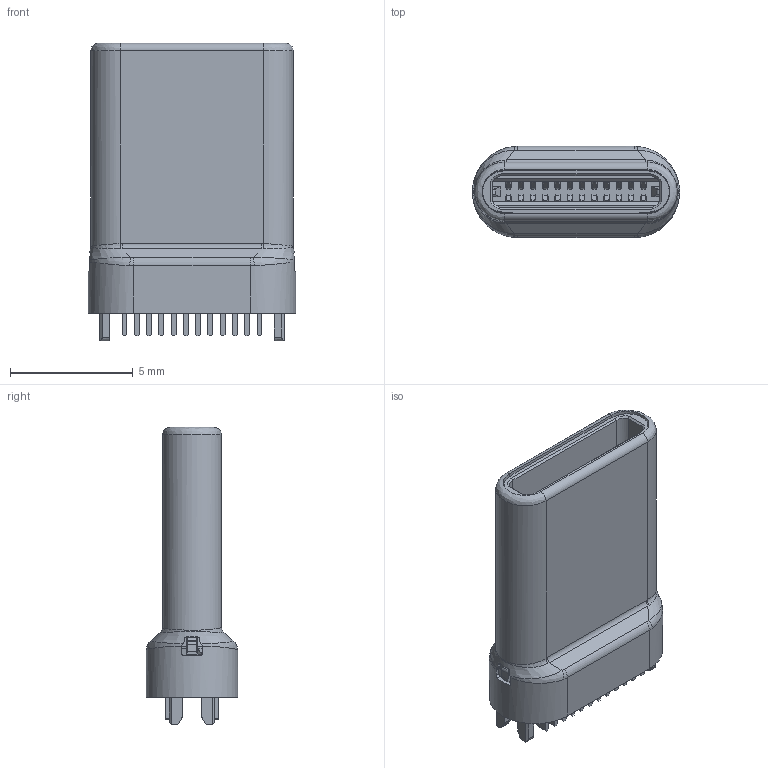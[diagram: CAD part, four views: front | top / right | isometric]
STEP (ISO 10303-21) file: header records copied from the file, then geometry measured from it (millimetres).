
FILE_DESCRIPTION (( 'STEP AP214' ), '1' );
FILE_NAME ('699C124-1A6-111 - EDAC USB Connector.STEP', '2021-01-19T17:44:34', ( '' ), ( '' ), 'SwSTEP 2.0', 'SolidWorks 2020', '' );
FILE_SCHEMA (( 'AUTOMOTIVE_DESIGN' ));
Length unit declared in the file: millimetre
Products named in the file (4): Shell 699C124-XA6-111; Insulator 699C124-XA6-111_Black; Contacts 699C124-XA6-111; 699C124-1A6-111 - EDAC USB Connector
Assembly tree (3 placements, depth 2):
  699C124-1A6-111 - EDAC USB Connector
    Insulator 699C124-XA6-111_Black
    Contacts 699C124-XA6-111
    Shell 699C124-XA6-111
Bounding box: 8.45 x 3.72 x 12.13 mm (x, y, z)
Volume: 177 mm3; surface area: 1467.2 mm2
Topology: 3 solids, 3 shells, 2005 faces, 5813 edges, 3781 vertices
Faces by surface type: plane 1449, cylinder 436, bspline 65, cone 55
Entity records: 71149 total; most frequent: CARTESIAN_POINT 17315, ORIENTED_EDGE 11622, DIRECTION 9895, EDGE_CURVE 5811, LINE 4447, VECTOR 4447, VERTEX_POINT 3781, AXIS2_PLACEMENT_3D 2724
